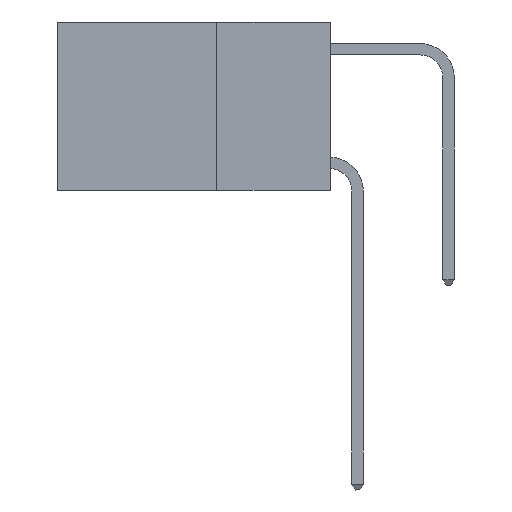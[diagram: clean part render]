
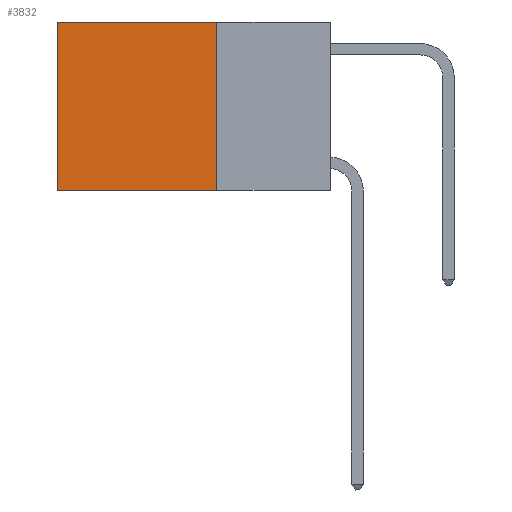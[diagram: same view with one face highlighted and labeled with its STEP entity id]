
A CAD part, left-side view. The second image highlights one B-rep face of the part: STEP entity #3832.
In plain terms, the highlighted planar face has unit normal (-1, 0, 0).
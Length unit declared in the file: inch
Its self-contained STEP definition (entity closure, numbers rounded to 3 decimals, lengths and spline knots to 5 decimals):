
#763 = VERTEX_POINT ( 'NONE', #3938 ) ;
#767 = VERTEX_POINT ( 'NONE', #1082 ) ;
#1082 = CARTESIAN_POINT ( 'NONE',  ( 0.2625, 0.6, 0. ) ) ;
#1771 = EDGE_CURVE ( 'NONE', #767, #8901, #5770, .T. ) ;
#1972 = DIRECTION ( 'NONE',  ( 0., 1., 0. ) ) ;
#1974 = LINE ( 'NONE', #2975, #11202 ) ;
#2115 = CARTESIAN_POINT ( 'NONE',  ( 0.2625, 0.25, -0.37 ) ) ;
#2240 = DIRECTION ( 'NONE',  ( 0., 1., 0. ) ) ;
#2333 = DIRECTION ( 'NONE',  ( 0., 0., -1. ) ) ;
#2373 = LINE ( 'NONE', #10523, #11781 ) ;
#2975 = CARTESIAN_POINT ( 'NONE',  ( 0.2625, 0.25, -0.37 ) ) ;
#3018 = VECTOR ( 'NONE', #6312, 39.37008 ) ;
#3763 = DIRECTION ( 'NONE',  ( 0., 0., -1. ) ) ;
#3832 = ADVANCED_FACE ( 'NONE', ( #10038 ), #8374, .F. ) ;
#3938 = CARTESIAN_POINT ( 'NONE',  ( 0.2625, 0.25, 0. ) ) ;
#5770 = LINE ( 'NONE', #6202, #3018 ) ;
#5847 = ORIENTED_EDGE ( 'NONE', *, *, #7742, .T. ) ;
#5898 = EDGE_CURVE ( 'NONE', #8570, #8901, #1974, .T. ) ;
#6156 = EDGE_CURVE ( 'NONE', #763, #8570, #11322, .T. ) ;
#6202 = CARTESIAN_POINT ( 'NONE',  ( 0.2625, 0.6, 0. ) ) ;
#6312 = DIRECTION ( 'NONE',  ( 0., 0., -1. ) ) ;
#6390 = AXIS2_PLACEMENT_3D ( 'NONE', #8333, #9297, #3763 ) ;
#6807 = EDGE_LOOP ( 'NONE', ( #11805, #7253, #10609, #5847 ) ) ;
#7170 = CARTESIAN_POINT ( 'NONE',  ( 0.2625, 0.6, -0.37 ) ) ;
#7253 = ORIENTED_EDGE ( 'NONE', *, *, #5898, .F. ) ;
#7742 = EDGE_CURVE ( 'NONE', #763, #767, #2373, .T. ) ;
#8333 = CARTESIAN_POINT ( 'NONE',  ( 0.2625, 0.25, 0. ) ) ;
#8374 = PLANE ( 'NONE',  #6390 ) ;
#8570 = VERTEX_POINT ( 'NONE', #2115 ) ;
#8667 = VECTOR ( 'NONE', #2333, 39.37008 ) ;
#8901 = VERTEX_POINT ( 'NONE', #7170 ) ;
#9297 = DIRECTION ( 'NONE',  ( 1., 0., 0. ) ) ;
#10038 = FACE_OUTER_BOUND ( 'NONE', #6807, .T. ) ;
#10523 = CARTESIAN_POINT ( 'NONE',  ( 0.2625, 0.25, 0. ) ) ;
#10609 = ORIENTED_EDGE ( 'NONE', *, *, #6156, .F. ) ;
#10644 = CARTESIAN_POINT ( 'NONE',  ( 0.2625, 0.25, 0. ) ) ;
#11202 = VECTOR ( 'NONE', #1972, 39.37008 ) ;
#11322 = LINE ( 'NONE', #10644, #8667 ) ;
#11781 = VECTOR ( 'NONE', #2240, 39.37008 ) ;
#11805 = ORIENTED_EDGE ( 'NONE', *, *, #1771, .T. ) ;
